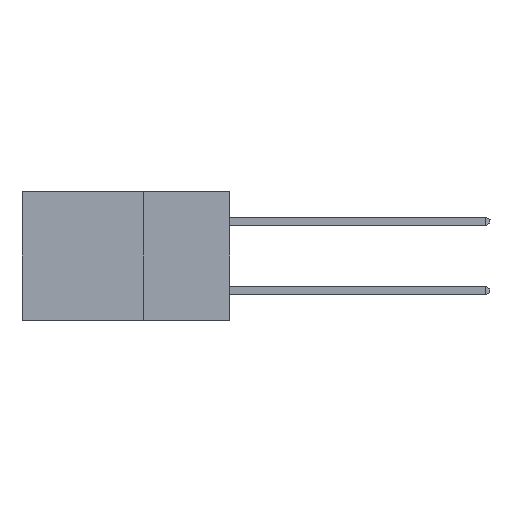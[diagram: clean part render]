
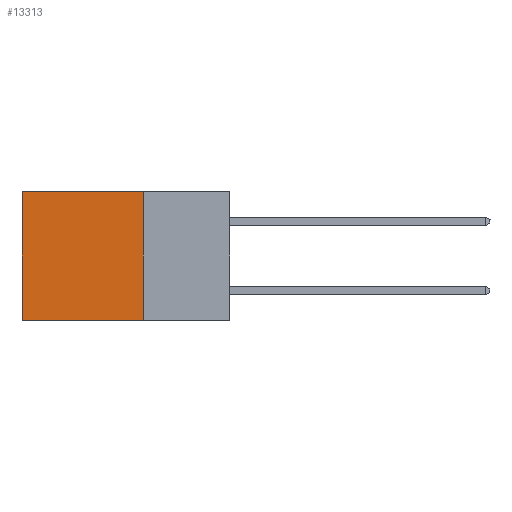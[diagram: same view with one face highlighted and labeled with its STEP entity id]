
A CAD part, left-side view. The second image highlights one B-rep face of the part: STEP entity #13313.
In plain terms, the highlighted planar face has unit normal (-1, 0, 0).
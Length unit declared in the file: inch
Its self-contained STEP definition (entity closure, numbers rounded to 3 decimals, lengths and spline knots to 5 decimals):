
#53 = VERTEX_POINT ( 'NONE', #10570 ) ;
#108 = LINE ( 'NONE', #1921, #4902 ) ;
#152 = ORIENTED_EDGE ( 'NONE', *, *, #18068, .F. ) ;
#1391 = CARTESIAN_POINT ( 'NONE',  ( 0.298, 0.25, -0.37 ) ) ;
#1921 = CARTESIAN_POINT ( 'NONE',  ( 0.298, 0.6, 0. ) ) ;
#1928 = CARTESIAN_POINT ( 'NONE',  ( 0.298, 0.25, 0. ) ) ;
#1997 = DIRECTION ( 'NONE',  ( 1., 0., 0. ) ) ;
#2533 = LINE ( 'NONE', #1391, #18755 ) ;
#3345 = DIRECTION ( 'NONE',  ( 0., 0., -1. ) ) ;
#3496 = CARTESIAN_POINT ( 'NONE',  ( 0.298, 0.25, 0. ) ) ;
#4278 = LINE ( 'NONE', #3496, #18720 ) ;
#4480 = EDGE_CURVE ( 'NONE', #53, #16805, #18693, .T. ) ;
#4580 = VERTEX_POINT ( 'NONE', #9967 ) ;
#4902 = VECTOR ( 'NONE', #3345, 39.37008 ) ;
#6359 = DIRECTION ( 'NONE',  ( 0., 1., 0. ) ) ;
#6761 = DIRECTION ( 'NONE',  ( 0., 0., -1. ) ) ;
#6902 = DIRECTION ( 'NONE',  ( 0., 0., -1. ) ) ;
#7359 = AXIS2_PLACEMENT_3D ( 'NONE', #1928, #1997, #6902 ) ;
#9617 = EDGE_LOOP ( 'NONE', ( #14403, #14988, #152, #13687 ) ) ;
#9967 = CARTESIAN_POINT ( 'NONE',  ( 0.298, 0.6, -0.37 ) ) ;
#10570 = CARTESIAN_POINT ( 'NONE',  ( 0.298, 0.25, 0. ) ) ;
#10752 = DIRECTION ( 'NONE',  ( 0., 1., 0. ) ) ;
#11668 = PLANE ( 'NONE',  #7359 ) ;
#12365 = EDGE_CURVE ( 'NONE', #17670, #4580, #2533, .T. ) ;
#13313 = ADVANCED_FACE ( 'NONE', ( #17992 ), #11668, .F. ) ;
#13687 = ORIENTED_EDGE ( 'NONE', *, *, #4480, .T. ) ;
#14403 = ORIENTED_EDGE ( 'NONE', *, *, #15785, .T. ) ;
#14988 = ORIENTED_EDGE ( 'NONE', *, *, #12365, .F. ) ;
#15455 = CARTESIAN_POINT ( 'NONE',  ( 0.298, 0.25, 0. ) ) ;
#15785 = EDGE_CURVE ( 'NONE', #16805, #4580, #108, .T. ) ;
#16805 = VERTEX_POINT ( 'NONE', #20974 ) ;
#17670 = VERTEX_POINT ( 'NONE', #20282 ) ;
#17972 = VECTOR ( 'NONE', #10752, 39.37008 ) ;
#17992 = FACE_OUTER_BOUND ( 'NONE', #9617, .T. ) ;
#18068 = EDGE_CURVE ( 'NONE', #53, #17670, #4278, .T. ) ;
#18693 = LINE ( 'NONE', #15455, #17972 ) ;
#18720 = VECTOR ( 'NONE', #6761, 39.37008 ) ;
#18755 = VECTOR ( 'NONE', #6359, 39.37008 ) ;
#20282 = CARTESIAN_POINT ( 'NONE',  ( 0.298, 0.25, -0.37 ) ) ;
#20974 = CARTESIAN_POINT ( 'NONE',  ( 0.298, 0.6, 0. ) ) ;
